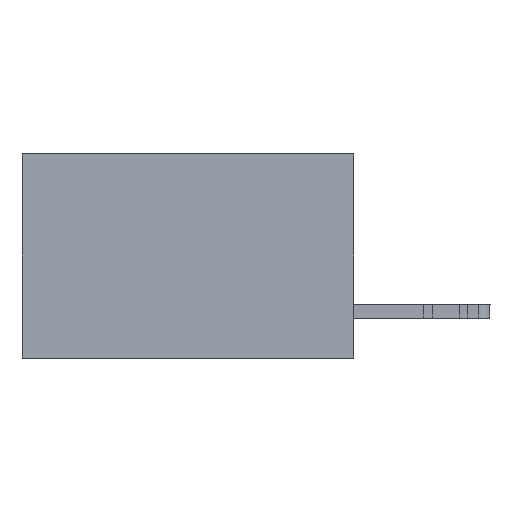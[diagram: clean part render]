
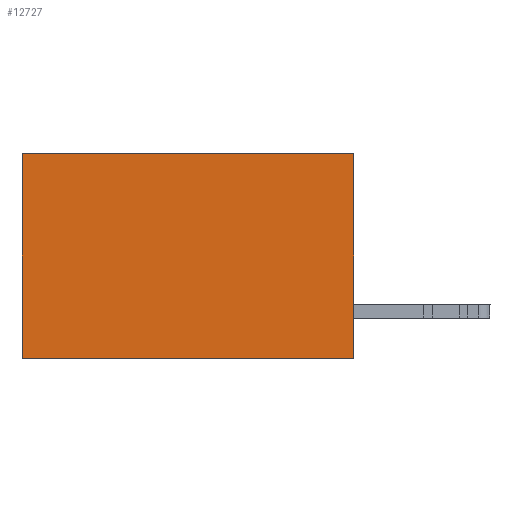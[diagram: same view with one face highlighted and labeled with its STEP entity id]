
A CAD part, left-side view. The second image highlights one B-rep face of the part: STEP entity #12727.
In plain terms, the highlighted planar face has unit normal (-1, 0, 0).
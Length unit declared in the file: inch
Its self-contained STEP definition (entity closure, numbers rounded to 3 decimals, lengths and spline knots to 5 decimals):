
#543 = CARTESIAN_POINT ( 'NONE',  ( 0.2875, 0., 0. ) ) ;
#1356 = DIRECTION ( 'NONE',  ( 0., 1., 0. ) ) ;
#1946 = DIRECTION ( 'NONE',  ( 0., 0., -1. ) ) ;
#2843 = ORIENTED_EDGE ( 'NONE', *, *, #21937, .F. ) ;
#4815 = LINE ( 'NONE', #36756, #22358 ) ;
#4973 = FACE_OUTER_BOUND ( 'NONE', #28275, .T. ) ;
#4992 = DIRECTION ( 'NONE',  ( 0., 0., -1. ) ) ;
#7766 = ORIENTED_EDGE ( 'NONE', *, *, #19880, .T. ) ;
#8118 = LINE ( 'NONE', #40073, #18010 ) ;
#9181 = CARTESIAN_POINT ( 'NONE',  ( 0.2875, 0.6, 0. ) ) ;
#10595 = VECTOR ( 'NONE', #4992, 39.37008 ) ;
#11760 = DIRECTION ( 'NONE',  ( 1., 0., 0. ) ) ;
#12727 = ADVANCED_FACE ( 'NONE', ( #4973 ), #36219, .F. ) ;
#14418 = CARTESIAN_POINT ( 'NONE',  ( 0.2875, 0.6, -0.37 ) ) ;
#18010 = VECTOR ( 'NONE', #1356, 39.37008 ) ;
#18290 = DIRECTION ( 'NONE',  ( 0., 0., -1. ) ) ;
#18451 = VERTEX_POINT ( 'NONE', #21445 ) ;
#19880 = EDGE_CURVE ( 'NONE', #32851, #18451, #8118, .T. ) ;
#21445 = CARTESIAN_POINT ( 'NONE',  ( 0.2875, 0.6, 0. ) ) ;
#21937 = EDGE_CURVE ( 'NONE', #32851, #26431, #27813, .T. ) ;
#22104 = DIRECTION ( 'NONE',  ( 0., 1., 0. ) ) ;
#22358 = VECTOR ( 'NONE', #22104, 39.37008 ) ;
#23555 = AXIS2_PLACEMENT_3D ( 'NONE', #32968, #11760, #18290 ) ;
#24923 = ORIENTED_EDGE ( 'NONE', *, *, #39819, .F. ) ;
#25467 = VERTEX_POINT ( 'NONE', #14418 ) ;
#26415 = VECTOR ( 'NONE', #1946, 39.37008 ) ;
#26431 = VERTEX_POINT ( 'NONE', #36700 ) ;
#27813 = LINE ( 'NONE', #37833, #26415 ) ;
#28275 = EDGE_LOOP ( 'NONE', ( #34312, #24923, #2843, #7766 ) ) ;
#32851 = VERTEX_POINT ( 'NONE', #543 ) ;
#32968 = CARTESIAN_POINT ( 'NONE',  ( 0.2875, 0., 0. ) ) ;
#34312 = ORIENTED_EDGE ( 'NONE', *, *, #42144, .T. ) ;
#35883 = LINE ( 'NONE', #9181, #10595 ) ;
#36219 = PLANE ( 'NONE',  #23555 ) ;
#36700 = CARTESIAN_POINT ( 'NONE',  ( 0.2875, 0., -0.37 ) ) ;
#36756 = CARTESIAN_POINT ( 'NONE',  ( 0.2875, 0., -0.37 ) ) ;
#37833 = CARTESIAN_POINT ( 'NONE',  ( 0.2875, 0., 0. ) ) ;
#39819 = EDGE_CURVE ( 'NONE', #26431, #25467, #4815, .T. ) ;
#40073 = CARTESIAN_POINT ( 'NONE',  ( 0.2875, 0., 0. ) ) ;
#42144 = EDGE_CURVE ( 'NONE', #18451, #25467, #35883, .T. ) ;
